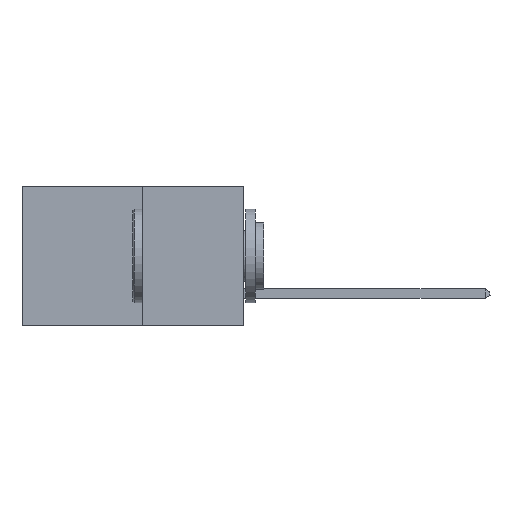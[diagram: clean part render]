
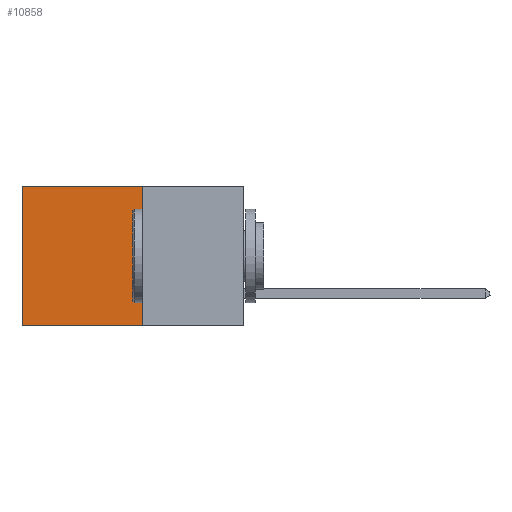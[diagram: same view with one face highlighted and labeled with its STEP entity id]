
A CAD part, left-side view. The second image highlights one B-rep face of the part: STEP entity #10858.
In plain terms, the highlighted planar face has unit normal (-1, 0, 0).
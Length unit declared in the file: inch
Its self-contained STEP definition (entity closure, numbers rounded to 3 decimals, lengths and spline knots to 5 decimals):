
#148 = EDGE_CURVE ( 'NONE', #1595, #13437, #11002, .T. ) ;
#157 = ORIENTED_EDGE ( 'NONE', *, *, #148, .T. ) ;
#212 = DIRECTION ( 'NONE',  ( 0., 1., 0. ) ) ;
#1595 = VERTEX_POINT ( 'NONE', #13806 ) ;
#1788 = CARTESIAN_POINT ( 'NONE',  ( 0.277, 0.27, -0.37 ) ) ;
#2133 = DIRECTION ( 'NONE',  ( 0., 1., 0. ) ) ;
#3136 = VERTEX_POINT ( 'NONE', #7628 ) ;
#3925 = CARTESIAN_POINT ( 'NONE',  ( 0.277, 0.27, -0.37 ) ) ;
#4941 = CARTESIAN_POINT ( 'NONE',  ( 0.277, 0.27, 0. ) ) ;
#5143 = DIRECTION ( 'NONE',  ( 0., 0., -1. ) ) ;
#5283 = ORIENTED_EDGE ( 'NONE', *, *, #7227, .T. ) ;
#5681 = ORIENTED_EDGE ( 'NONE', *, *, #11981, .F. ) ;
#7227 = EDGE_CURVE ( 'NONE', #13437, #3136, #13089, .T. ) ;
#7628 = CARTESIAN_POINT ( 'NONE',  ( 0.277, 0.59, -0.37 ) ) ;
#7813 = VECTOR ( 'NONE', #2133, 39.37008 ) ;
#8220 = VECTOR ( 'NONE', #212, 39.37008 ) ;
#8529 = AXIS2_PLACEMENT_3D ( 'NONE', #3925, #12312, #5143 ) ;
#9025 = DIRECTION ( 'NONE',  ( 0., 0., -1. ) ) ;
#9060 = EDGE_LOOP ( 'NONE', ( #5283, #5681, #9621, #157 ) ) ;
#9497 = CARTESIAN_POINT ( 'NONE',  ( 0.277, 0.59, 0. ) ) ;
#9591 = FACE_OUTER_BOUND ( 'NONE', #9060, .T. ) ;
#9621 = ORIENTED_EDGE ( 'NONE', *, *, #14487, .F. ) ;
#10858 = ADVANCED_FACE ( 'NONE', ( #9591 ), #11145, .F. ) ;
#11002 = LINE ( 'NONE', #4941, #7813 ) ;
#11145 = PLANE ( 'NONE',  #8529 ) ;
#11487 = DIRECTION ( 'NONE',  ( 0., 0., -1. ) ) ;
#11544 = CARTESIAN_POINT ( 'NONE',  ( 0.277, 0.59, -0.37 ) ) ;
#11981 = EDGE_CURVE ( 'NONE', #14916, #3136, #15253, .T. ) ;
#12053 = VECTOR ( 'NONE', #9025, 39.37008 ) ;
#12226 = CARTESIAN_POINT ( 'NONE',  ( 0.277, 0.27, -0.37 ) ) ;
#12312 = DIRECTION ( 'NONE',  ( 1., 0., 0. ) ) ;
#12703 = VECTOR ( 'NONE', #11487, 39.37008 ) ;
#13089 = LINE ( 'NONE', #11544, #12703 ) ;
#13437 = VERTEX_POINT ( 'NONE', #9497 ) ;
#13806 = CARTESIAN_POINT ( 'NONE',  ( 0.277, 0.27, 0. ) ) ;
#14487 = EDGE_CURVE ( 'NONE', #1595, #14916, #15154, .T. ) ;
#14916 = VERTEX_POINT ( 'NONE', #15178 ) ;
#15154 = LINE ( 'NONE', #1788, #12053 ) ;
#15178 = CARTESIAN_POINT ( 'NONE',  ( 0.277, 0.27, -0.37 ) ) ;
#15253 = LINE ( 'NONE', #12226, #8220 ) ;
